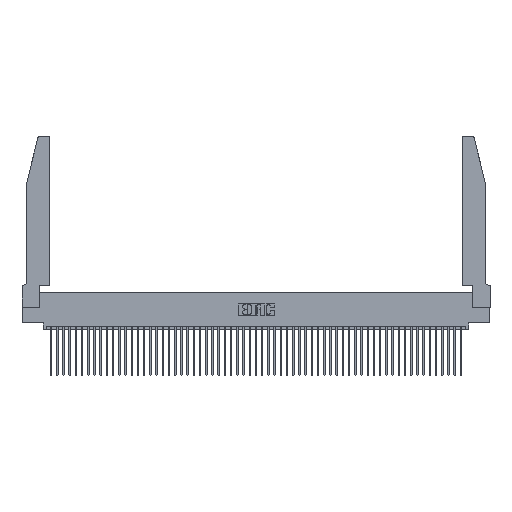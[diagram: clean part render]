
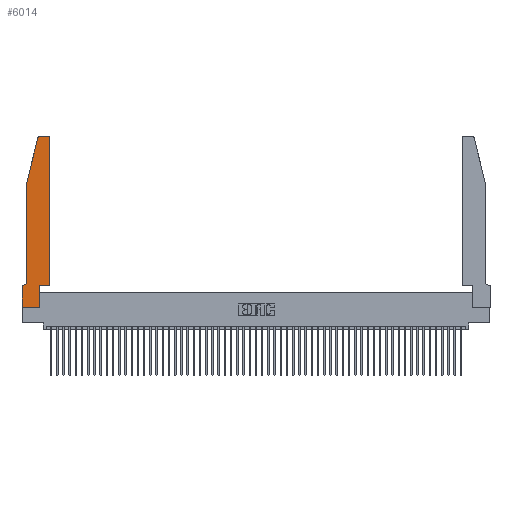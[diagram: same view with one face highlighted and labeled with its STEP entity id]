
A CAD part, top view. The second image highlights one B-rep face of the part: STEP entity #6014.
In plain terms, the highlighted planar face has unit normal (0, 0, 1).
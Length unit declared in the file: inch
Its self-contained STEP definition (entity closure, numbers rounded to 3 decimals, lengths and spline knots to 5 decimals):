
#764 = LINE ( 'NONE', #48379, #44000 ) ;
#1022 = DIRECTION ( 'NONE',  ( 0., -1., 0. ) ) ;
#1516 = FACE_OUTER_BOUND ( 'NONE', #32979, .T. ) ;
#1671 = CARTESIAN_POINT ( 'NONE',  ( 0.284, 2.72, 0.37 ) ) ;
#3206 = CARTESIAN_POINT ( 'NONE',  ( 0.4505, 0.35, 0.37 ) ) ;
#3240 = LINE ( 'NONE', #3206, #13108 ) ;
#3298 = ORIENTED_EDGE ( 'NONE', *, *, #15013, .T. ) ;
#3369 = VERTEX_POINT ( 'NONE', #41700 ) ;
#3602 = ORIENTED_EDGE ( 'NONE', *, *, #24308, .T. ) ;
#4260 = CARTESIAN_POINT ( 'NONE',  ( 0.0755, 0.42, 0.37 ) ) ;
#4352 = CARTESIAN_POINT ( 'NONE',  ( 0.0755, 0.35, 0.37 ) ) ;
#4458 = ORIENTED_EDGE ( 'NONE', *, *, #37037, .T. ) ;
#4472 = DIRECTION ( 'NONE',  ( 0., 1., 0. ) ) ;
#4981 = CARTESIAN_POINT ( 'NONE',  ( 0.0755, 2., 0.37 ) ) ;
#5047 = CARTESIAN_POINT ( 'NONE',  ( 0.4505, 0.35, 0.37 ) ) ;
#5869 = VECTOR ( 'NONE', #17075, 39.37008 ) ;
#5895 = DIRECTION ( 'NONE',  ( 1., 0., 0. ) ) ;
#6014 = ADVANCED_FACE ( 'NONE', ( #1516 ), #38244, .T. ) ;
#6451 = EDGE_CURVE ( 'NONE', #3369, #49526, #3240, .T. ) ;
#7189 = LINE ( 'NONE', #4352, #5869 ) ;
#7531 = CARTESIAN_POINT ( 'NONE',  ( 0.4205, 2.72, 0.37 ) ) ;
#8671 = CARTESIAN_POINT ( 'NONE',  ( 0.4505, 0.35, 0.37 ) ) ;
#9221 = DIRECTION ( 'NONE',  ( -0.239, -0.971, 0. ) ) ;
#11659 = DIRECTION ( 'NONE',  ( 1., 0., 0. ) ) ;
#11759 = DIRECTION ( 'NONE',  ( 1., 0., 0. ) ) ;
#11819 = CARTESIAN_POINT ( 'NONE',  ( 0., 0., 0.37 ) ) ;
#11832 = ORIENTED_EDGE ( 'NONE', *, *, #52122, .T. ) ;
#12036 = LINE ( 'NONE', #4981, #32997 ) ;
#12130 = ORIENTED_EDGE ( 'NONE', *, *, #35176, .T. ) ;
#13077 = CARTESIAN_POINT ( 'NONE',  ( 0.4205, 2.75, 0.37 ) ) ;
#13108 = VECTOR ( 'NONE', #11659, 39.37008 ) ;
#13161 = EDGE_CURVE ( 'NONE', #45235, #3369, #53193, .T. ) ;
#13307 = CARTESIAN_POINT ( 'NONE',  ( 0., 0., 0.37 ) ) ;
#13531 = CARTESIAN_POINT ( 'NONE',  ( 0., 0., 0.37 ) ) ;
#13564 = VERTEX_POINT ( 'NONE', #20123 ) ;
#13851 = LINE ( 'NONE', #11819, #33468 ) ;
#13857 = CARTESIAN_POINT ( 'NONE',  ( 0., 0.35, 0.37 ) ) ;
#13911 = LINE ( 'NONE', #22844, #45926 ) ;
#14009 = VERTEX_POINT ( 'NONE', #48297 ) ;
#14241 = AXIS2_PLACEMENT_3D ( 'NONE', #7531, #36836, #11759 ) ;
#15013 = EDGE_CURVE ( 'NONE', #30431, #45235, #13851, .T. ) ;
#16056 = DIRECTION ( 'NONE',  ( 1., 0., 0. ) ) ;
#16828 = AXIS2_PLACEMENT_3D ( 'NONE', #24589, #53703, #28769 ) ;
#17075 = DIRECTION ( 'NONE',  ( -1., 0., 0. ) ) ;
#17369 = EDGE_CURVE ( 'NONE', #49526, #42637, #35267, .T. ) ;
#17769 = DIRECTION ( 'NONE',  ( 0., 1., 0. ) ) ;
#20123 = CARTESIAN_POINT ( 'NONE',  ( 0.25487, 2.72718, 0.37 ) ) ;
#20471 = CARTESIAN_POINT ( 'NONE',  ( 0.4505, 2.72, 0.37 ) ) ;
#21789 = ORIENTED_EDGE ( 'NONE', *, *, #17369, .T. ) ;
#21807 = AXIS2_PLACEMENT_3D ( 'NONE', #34023, #25647, #42436 ) ;
#22121 = VERTEX_POINT ( 'NONE', #41738 ) ;
#22597 = VECTOR ( 'NONE', #4472, 39.37008 ) ;
#22689 = ORIENTED_EDGE ( 'NONE', *, *, #39501, .T. ) ;
#22691 = CIRCLE ( 'NONE', #29297, 0.03 ) ;
#22844 = CARTESIAN_POINT ( 'NONE',  ( 0.0755, 2., 0.37 ) ) ;
#23116 = EDGE_CURVE ( 'NONE', #25553, #35856, #764, .T. ) ;
#23193 = VERTEX_POINT ( 'NONE', #13857 ) ;
#23288 = EDGE_CURVE ( 'NONE', #22121, #36918, #13911, .T. ) ;
#23315 = CIRCLE ( 'NONE', #14241, 0.03 ) ;
#23341 = CARTESIAN_POINT ( 'NONE',  ( 0.2865, 0., 0.37 ) ) ;
#24240 = ORIENTED_EDGE ( 'NONE', *, *, #6451, .T. ) ;
#24308 = EDGE_CURVE ( 'NONE', #14009, #23193, #7189, .T. ) ;
#24488 = CIRCLE ( 'NONE', #16828, 0.07 ) ;
#24589 = CARTESIAN_POINT ( 'NONE',  ( 0.0055, 0.42, 0.37 ) ) ;
#25553 = VERTEX_POINT ( 'NONE', #13077 ) ;
#25647 = DIRECTION ( 'NONE',  ( 0., 0., 1. ) ) ;
#27025 = DIRECTION ( 'NONE',  ( 0., -1., 0. ) ) ;
#27368 = ORIENTED_EDGE ( 'NONE', *, *, #23288, .T. ) ;
#28596 = VECTOR ( 'NONE', #1022, 39.37008 ) ;
#28769 = DIRECTION ( 'NONE',  ( -1., 0., 0. ) ) ;
#29297 = AXIS2_PLACEMENT_3D ( 'NONE', #1671, #31017, #5895 ) ;
#29595 = CARTESIAN_POINT ( 'NONE',  ( 0.2865, 0.35, 0.37 ) ) ;
#30431 = VERTEX_POINT ( 'NONE', #13307 ) ;
#31017 = DIRECTION ( 'NONE',  ( 0., 0., 1. ) ) ;
#32979 = EDGE_LOOP ( 'NONE', ( #34408, #12130, #4458, #27368, #22689, #3602, #11832, #3298, #34273, #24240, #21789, #47186 ) ) ;
#32997 = VECTOR ( 'NONE', #9221, 39.37008 ) ;
#33468 = VECTOR ( 'NONE', #16056, 39.37008 ) ;
#33954 = VECTOR ( 'NONE', #17769, 39.37008 ) ;
#34023 = CARTESIAN_POINT ( 'NONE',  ( 0., 0.35, 0.37 ) ) ;
#34273 = ORIENTED_EDGE ( 'NONE', *, *, #13161, .T. ) ;
#34408 = ORIENTED_EDGE ( 'NONE', *, *, #23116, .T. ) ;
#35176 = EDGE_CURVE ( 'NONE', #35856, #13564, #22691, .T. ) ;
#35267 = LINE ( 'NONE', #5047, #33954 ) ;
#35412 = EDGE_CURVE ( 'NONE', #42637, #25553, #23315, .T. ) ;
#35856 = VERTEX_POINT ( 'NONE', #43547 ) ;
#36836 = DIRECTION ( 'NONE',  ( 0., 0., 1. ) ) ;
#36918 = VERTEX_POINT ( 'NONE', #4260 ) ;
#37037 = EDGE_CURVE ( 'NONE', #13564, #22121, #12036, .T. ) ;
#38244 = PLANE ( 'NONE',  #21807 ) ;
#39501 = EDGE_CURVE ( 'NONE', #36918, #14009, #24488, .T. ) ;
#41027 = LINE ( 'NONE', #13531, #28596 ) ;
#41700 = CARTESIAN_POINT ( 'NONE',  ( 0.2865, 0.35, 0.37 ) ) ;
#41738 = CARTESIAN_POINT ( 'NONE',  ( 0.0755, 2., 0.37 ) ) ;
#42436 = DIRECTION ( 'NONE',  ( 1., 0., 0. ) ) ;
#42637 = VERTEX_POINT ( 'NONE', #20471 ) ;
#43547 = CARTESIAN_POINT ( 'NONE',  ( 0.284, 2.75, 0.37 ) ) ;
#44000 = VECTOR ( 'NONE', #44195, 39.37008 ) ;
#44195 = DIRECTION ( 'NONE',  ( -1., 0., 0. ) ) ;
#45235 = VERTEX_POINT ( 'NONE', #23341 ) ;
#45926 = VECTOR ( 'NONE', #27025, 39.37008 ) ;
#47186 = ORIENTED_EDGE ( 'NONE', *, *, #35412, .T. ) ;
#48297 = CARTESIAN_POINT ( 'NONE',  ( 0.0055, 0.35, 0.37 ) ) ;
#48379 = CARTESIAN_POINT ( 'NONE',  ( 0.2605, 2.75, 0.37 ) ) ;
#49526 = VERTEX_POINT ( 'NONE', #8671 ) ;
#52122 = EDGE_CURVE ( 'NONE', #23193, #30431, #41027, .T. ) ;
#53193 = LINE ( 'NONE', #29595, #22597 ) ;
#53703 = DIRECTION ( 'NONE',  ( 0., 0., -1. ) ) ;
